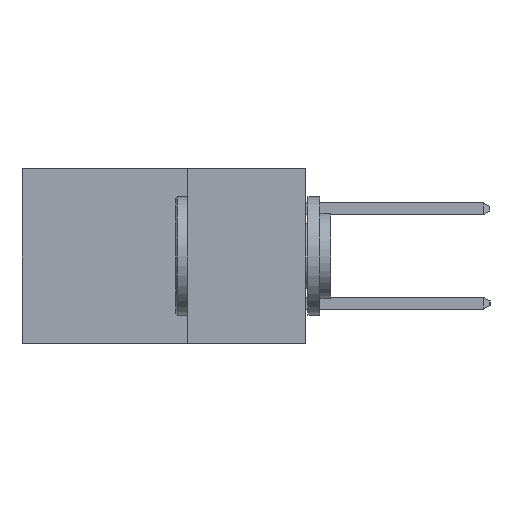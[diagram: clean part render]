
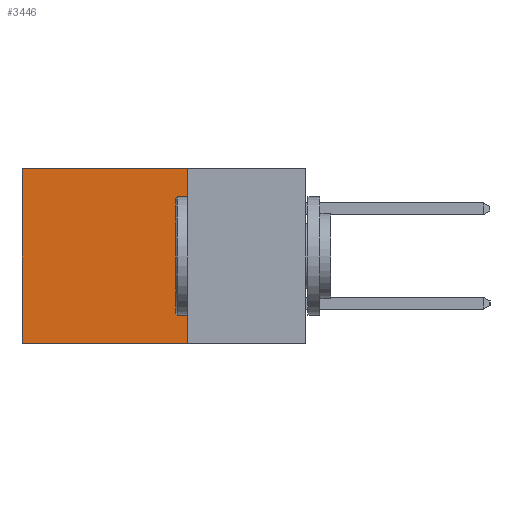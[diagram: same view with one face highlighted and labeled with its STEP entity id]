
A CAD part, left-side view. The second image highlights one B-rep face of the part: STEP entity #3446.
In plain terms, the highlighted planar face has unit normal (-1, 0, 0).
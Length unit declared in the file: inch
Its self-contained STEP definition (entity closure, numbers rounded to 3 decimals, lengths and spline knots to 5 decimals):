
#825 = ORIENTED_EDGE ( 'NONE', *, *, #5197, .F. ) ;
#832 = EDGE_CURVE ( 'NONE', #14191, #15656, #17501, .T. ) ;
#1893 = DIRECTION ( 'NONE',  ( 0., 0., -1. ) ) ;
#1982 = DIRECTION ( 'NONE',  ( 1., 0., 0. ) ) ;
#2022 = ORIENTED_EDGE ( 'NONE', *, *, #14958, .T. ) ;
#2200 = CARTESIAN_POINT ( 'NONE',  ( 0.2615, 0.6, -0.37 ) ) ;
#2248 = CARTESIAN_POINT ( 'NONE',  ( 0.2615, 0.25, -0.37 ) ) ;
#2271 = PLANE ( 'NONE',  #4095 ) ;
#2718 = EDGE_LOOP ( 'NONE', ( #2022, #825, #9121, #12612 ) ) ;
#2771 = DIRECTION ( 'NONE',  ( 0., 0., -1. ) ) ;
#3446 = ADVANCED_FACE ( 'NONE', ( #18456 ), #2271, .F. ) ;
#3584 = VERTEX_POINT ( 'NONE', #9906 ) ;
#4085 = LINE ( 'NONE', #2200, #7526 ) ;
#4095 = AXIS2_PLACEMENT_3D ( 'NONE', #2248, #1982, #1893 ) ;
#4285 = LINE ( 'NONE', #12772, #7724 ) ;
#5197 = EDGE_CURVE ( 'NONE', #15656, #10421, #4285, .T. ) ;
#5734 = LINE ( 'NONE', #11582, #12732 ) ;
#7526 = VECTOR ( 'NONE', #12236, 39.37008 ) ;
#7724 = VECTOR ( 'NONE', #12351, 39.37008 ) ;
#7915 = CARTESIAN_POINT ( 'NONE',  ( 0.2615, 0.6, -0.37 ) ) ;
#8573 = CARTESIAN_POINT ( 'NONE',  ( 0.2615, 0.25, -0.37 ) ) ;
#9121 = ORIENTED_EDGE ( 'NONE', *, *, #832, .F. ) ;
#9328 = EDGE_CURVE ( 'NONE', #14191, #3584, #5734, .T. ) ;
#9906 = CARTESIAN_POINT ( 'NONE',  ( 0.2615, 0.6, 0. ) ) ;
#10211 = DIRECTION ( 'NONE',  ( 0., 1., 0. ) ) ;
#10421 = VERTEX_POINT ( 'NONE', #7915 ) ;
#11582 = CARTESIAN_POINT ( 'NONE',  ( 0.2615, 0.25, 0. ) ) ;
#12236 = DIRECTION ( 'NONE',  ( 0., 0., -1. ) ) ;
#12351 = DIRECTION ( 'NONE',  ( 0., 1., 0. ) ) ;
#12612 = ORIENTED_EDGE ( 'NONE', *, *, #9328, .T. ) ;
#12732 = VECTOR ( 'NONE', #10211, 39.37008 ) ;
#12772 = CARTESIAN_POINT ( 'NONE',  ( 0.2615, 0.25, -0.37 ) ) ;
#13644 = CARTESIAN_POINT ( 'NONE',  ( 0.2615, 0.25, -0.37 ) ) ;
#14191 = VERTEX_POINT ( 'NONE', #14923 ) ;
#14923 = CARTESIAN_POINT ( 'NONE',  ( 0.2615, 0.25, 0. ) ) ;
#14958 = EDGE_CURVE ( 'NONE', #3584, #10421, #4085, .T. ) ;
#15656 = VERTEX_POINT ( 'NONE', #13644 ) ;
#17072 = VECTOR ( 'NONE', #2771, 39.37008 ) ;
#17501 = LINE ( 'NONE', #8573, #17072 ) ;
#18456 = FACE_OUTER_BOUND ( 'NONE', #2718, .T. ) ;
